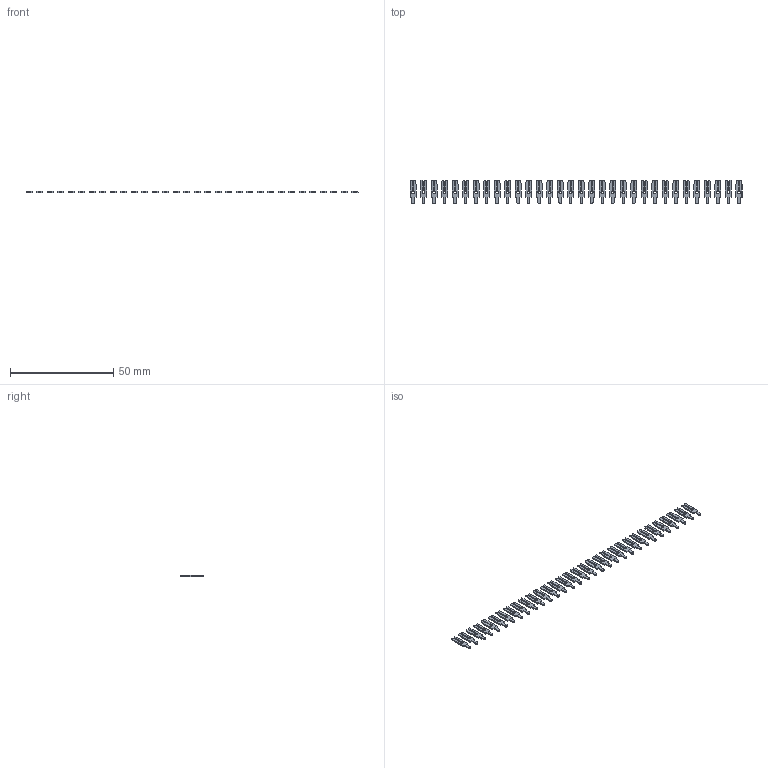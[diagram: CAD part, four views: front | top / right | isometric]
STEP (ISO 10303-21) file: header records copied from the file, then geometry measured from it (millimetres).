
FILE_DESCRIPTION (( 'STEP AP203' ), '1' );
FILE_NAME ('103-032-250-200.STEP', '2020-04-09T20:55:23', ( '' ), ( '' ), 'SwSTEP 2.0', 'SolidWorks 2016', '' );
FILE_SCHEMA (( 'CONFIG_CONTROL_DESIGN' ));
Length unit declared in the file: inch
Products named in the file (2): 103-032-250-200; 100-290-001_100-290-250
Assembly tree (32 placements, depth 2):
  103-032-250-200
    100-290-001_100-290-250  x32
Bounding box: 160.4 x 11.48 x 0.66 mm (x, y, z)
Volume: 499.4 mm3; surface area: 2347.2 mm2
Topology: 32 solids, 32 shells, 768 faces, 2112 edges, 1408 vertices
Faces by surface type: plane 640, cylinder 128
Entity records: 1950 total; most frequent: DIRECTION 188, CARTESIAN_POINT 181, ORIENTED_EDGE 132, CALENDAR_DATE 74, DATE_AND_TIME 74, COORDINATED_UNIVERSAL_TIME_OFFSET 74, LOCAL_TIME 74, AXIS2_PLACEMENT_3D 67
